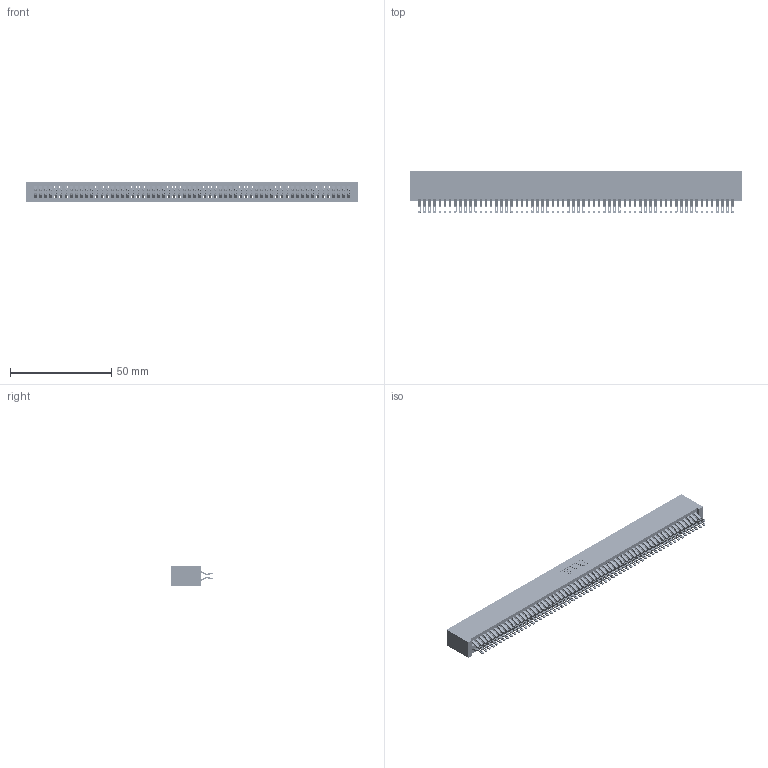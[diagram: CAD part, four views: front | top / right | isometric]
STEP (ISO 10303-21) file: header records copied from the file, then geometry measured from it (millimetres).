
FILE_DESCRIPTION (( 'STEP AP203' ), '1' );
FILE_NAME ('395-124-555-201.STEP', '2018-12-04T00:41:41', ( '' ), ( '' ), 'SwSTEP 2.0', 'SolidWorks 2016', '' );
FILE_SCHEMA (( 'CONFIG_CONTROL_DESIGN' ));
Length unit declared in the file: inch
Products named in the file (3): 395-124-555-201; 345 Part_No Mounting Lugs; 345-292-001_555 Tail
Assembly tree (125 placements, depth 2):
  395-124-555-201
    345 Part_No Mounting Lugs
    345-292-001_555 Tail  x124
Bounding box: 164.08 x 21.13 x 9.4 mm (x, y, z)
Volume: 17100.5 mm3; surface area: 27219 mm2
Topology: 125 solids, 125 shells, 7062 faces, 22265 edges, 14842 vertices
Faces by surface type: plane 3920, cylinder 3142
Entity records: 46003 total; most frequent: CARTESIAN_POINT 7726, ORIENTED_EDGE 7630, DIRECTION 6751, EDGE_CURVE 3815, LINE 3423, VECTOR 3423, VERTEX_POINT 2542, AXIS2_PLACEMENT_3D 1664
